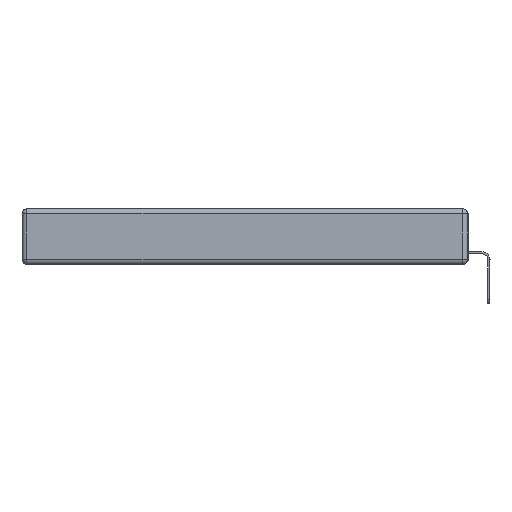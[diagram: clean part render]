
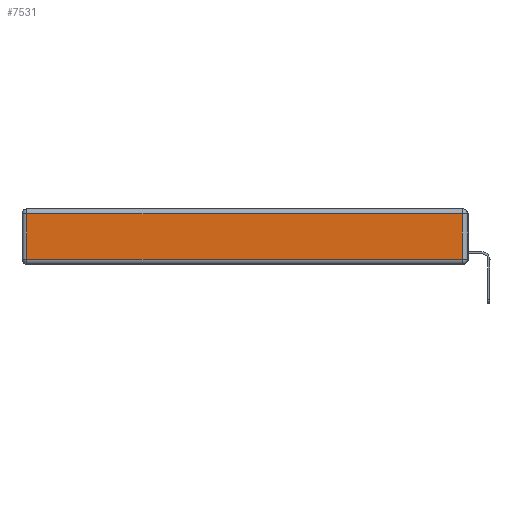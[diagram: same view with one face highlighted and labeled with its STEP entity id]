
A CAD part, left-side view. The second image highlights one B-rep face of the part: STEP entity #7531.
In plain terms, the highlighted planar face has unit normal (-1, 0, 0).
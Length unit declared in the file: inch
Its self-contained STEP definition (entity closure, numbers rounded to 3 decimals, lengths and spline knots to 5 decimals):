
#113 = LINE ( 'NONE', #10110, #18435 ) ;
#251 = CARTESIAN_POINT ( 'NONE',  ( 0., 2.72, -0.313 ) ) ;
#705 = EDGE_LOOP ( 'NONE', ( #6166, #9057, #4004, #23931 ) ) ;
#2614 = CARTESIAN_POINT ( 'NONE',  ( 0., 0., -0.343 ) ) ;
#2640 = FACE_OUTER_BOUND ( 'NONE', #705, .T. ) ;
#2931 = VERTEX_POINT ( 'NONE', #3275 ) ;
#3275 = CARTESIAN_POINT ( 'NONE',  ( 0., 2.72, -0.03 ) ) ;
#4004 = ORIENTED_EDGE ( 'NONE', *, *, #14304, .T. ) ;
#4479 = EDGE_CURVE ( 'NONE', #25232, #14855, #113, .T. ) ;
#4810 = PLANE ( 'NONE',  #15357 ) ;
#5257 = LINE ( 'NONE', #14515, #15069 ) ;
#5928 = DIRECTION ( 'NONE',  ( 0., 0., 1. ) ) ;
#6166 = ORIENTED_EDGE ( 'NONE', *, *, #24696, .T. ) ;
#7523 = VECTOR ( 'NONE', #21393, 39.37008 ) ;
#7531 = ADVANCED_FACE ( 'NONE', ( #2640 ), #4810, .T. ) ;
#9057 = ORIENTED_EDGE ( 'NONE', *, *, #4479, .T. ) ;
#10110 = CARTESIAN_POINT ( 'NONE',  ( 0., 0.03, -0.343 ) ) ;
#11036 = CARTESIAN_POINT ( 'NONE',  ( 0., 0., -0.313 ) ) ;
#13402 = VECTOR ( 'NONE', #23651, 39.37008 ) ;
#14304 = EDGE_CURVE ( 'NONE', #14855, #2931, #21918, .T. ) ;
#14515 = CARTESIAN_POINT ( 'NONE',  ( 0., 2.72, -0.343 ) ) ;
#14855 = VERTEX_POINT ( 'NONE', #18849 ) ;
#15069 = VECTOR ( 'NONE', #16459, 39.37008 ) ;
#15192 = CARTESIAN_POINT ( 'NONE',  ( 0., 0.03, -0.313 ) ) ;
#15357 = AXIS2_PLACEMENT_3D ( 'NONE', #2614, #23472, #19339 ) ;
#16459 = DIRECTION ( 'NONE',  ( 0., 0., -1. ) ) ;
#18435 = VECTOR ( 'NONE', #5928, 39.37008 ) ;
#18849 = CARTESIAN_POINT ( 'NONE',  ( 0., 0.03, -0.03 ) ) ;
#19339 = DIRECTION ( 'NONE',  ( 0., 0., 1. ) ) ;
#21393 = DIRECTION ( 'NONE',  ( 0., 1., 0. ) ) ;
#21918 = LINE ( 'NONE', #25475, #7523 ) ;
#23472 = DIRECTION ( 'NONE',  ( -1., 0., 0. ) ) ;
#23651 = DIRECTION ( 'NONE',  ( 0., -1., 0. ) ) ;
#23931 = ORIENTED_EDGE ( 'NONE', *, *, #24381, .T. ) ;
#24262 = LINE ( 'NONE', #11036, #13402 ) ;
#24381 = EDGE_CURVE ( 'NONE', #2931, #24515, #5257, .T. ) ;
#24515 = VERTEX_POINT ( 'NONE', #251 ) ;
#24696 = EDGE_CURVE ( 'NONE', #24515, #25232, #24262, .T. ) ;
#25232 = VERTEX_POINT ( 'NONE', #15192 ) ;
#25475 = CARTESIAN_POINT ( 'NONE',  ( 0., 2.75, -0.03 ) ) ;
